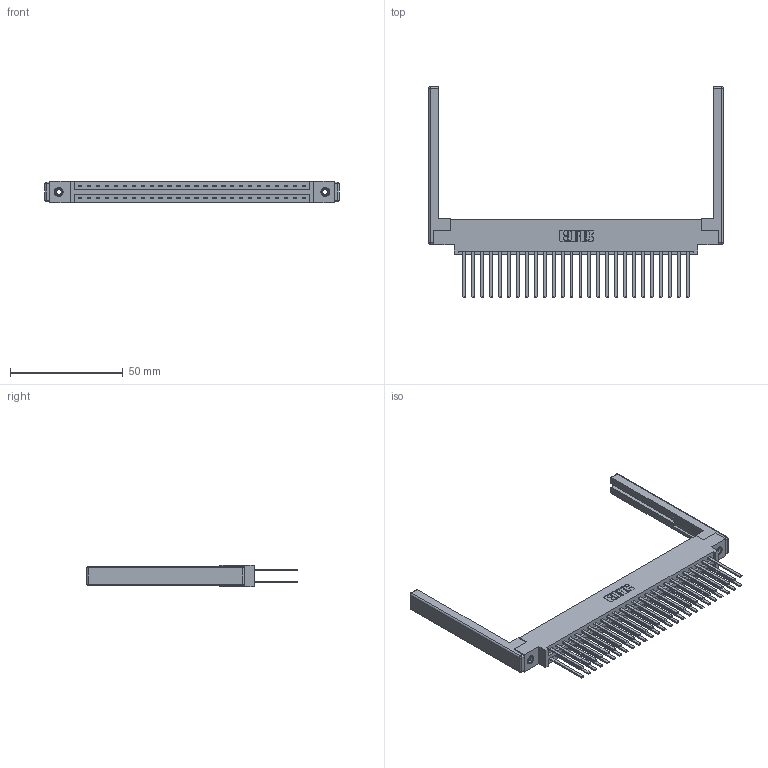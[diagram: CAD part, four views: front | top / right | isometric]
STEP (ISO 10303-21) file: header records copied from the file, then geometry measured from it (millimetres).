
FILE_DESCRIPTION (( 'STEP AP203' ), '1' );
FILE_NAME ('387-052-544-868.STEP', '2019-10-19T03:38:27', ( '' ), ( '' ), 'SwSTEP 2.0', 'SolidWorks 2016', '' );
FILE_SCHEMA (( 'CONFIG_CONTROL_DESIGN' ));
Length unit declared in the file: inch
Products named in the file (5): 337 Part_0.170 Offset - 0.156 Dia-TI; 345-292-001_345-293-144; 307-220-068; 345-250-001_345-250-001-102; 387-052-544-868
Assembly tree (57 placements, depth 2):
  387-052-544-868
    337 Part_0.170 Offset - 0.156 Dia-TI
    345-292-001_345-293-144  x52
    345-250-001_345-250-001-102  x2
    307-220-068  x2
Bounding box: 130.45 x 93.35 x 9.4 mm (x, y, z)
Volume: 18531.6 mm3; surface area: 22361 mm2
Topology: 57 solids, 57 shells, 2768 faces, 8149 edges, 5342 vertices
Faces by surface type: plane 1930, cylinder 814, cone 12, sphere 8, torus 4
Entity records: 24936 total; most frequent: CARTESIAN_POINT 4179, ORIENTED_EDGE 4104, DIRECTION 3650, EDGE_CURVE 2052, VECTOR 1878, LINE 1878, VERTEX_POINT 1358, AXIS2_PLACEMENT_3D 886
